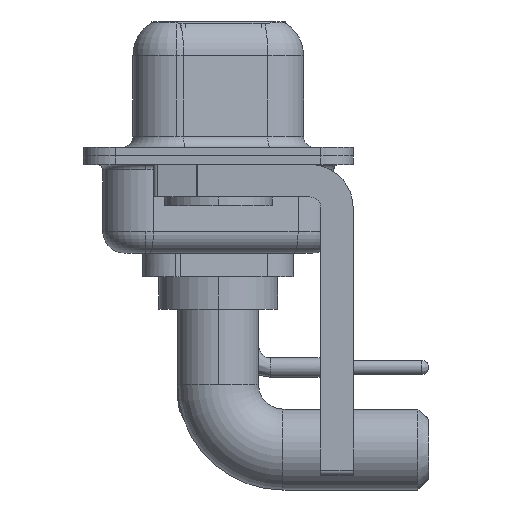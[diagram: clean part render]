
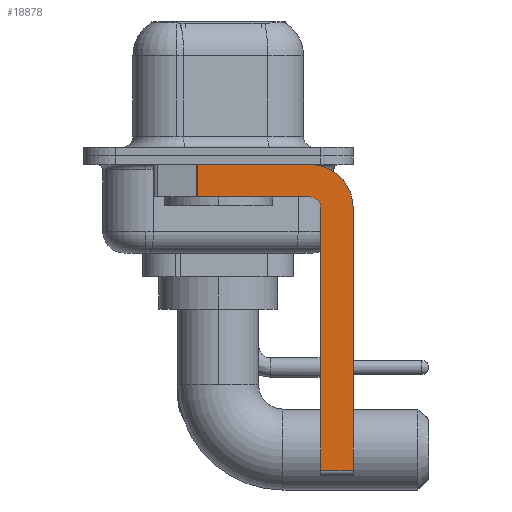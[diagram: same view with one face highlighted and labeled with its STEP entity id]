
A CAD part, left-side view. The second image highlights one B-rep face of the part: STEP entity #18878.
In plain terms, the highlighted planar face has unit normal (-1, 0, 0).
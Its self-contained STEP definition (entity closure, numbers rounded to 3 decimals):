
#360 = CARTESIAN_POINT ( 'NONE',  ( -2.9, -4.25, -0.4 ) ) ;
#599 = CARTESIAN_POINT ( 'NONE',  ( -2.9, -4.25, -1.9 ) ) ;
#852 = DIRECTION ( 'NONE',  ( 0., 0., 1. ) ) ;
#1183 = LINE ( 'NONE', #599, #2556 ) ;
#1853 = DIRECTION ( 'NONE',  ( 1., 0., 0. ) ) ;
#1893 = DIRECTION ( 'NONE',  ( -1., 0., 0. ) ) ;
#1949 = LINE ( 'NONE', #15132, #15423 ) ;
#2354 = EDGE_LOOP ( 'NONE', ( #16925, #16389, #22861, #15963, #22969, #20621, #24127, #7540 ) ) ;
#2556 = VECTOR ( 'NONE', #23903, 1000. ) ;
#2571 = VERTEX_POINT ( 'NONE', #15135 ) ;
#3588 = VECTOR ( 'NONE', #19046, 1000. ) ;
#4960 = VERTEX_POINT ( 'NONE', #17312 ) ;
#4984 = VERTEX_POINT ( 'NONE', #20901 ) ;
#5186 = LINE ( 'NONE', #14515, #7699 ) ;
#5392 = EDGE_CURVE ( 'NONE', #17463, #19019, #10856, .T. ) ;
#5721 = CARTESIAN_POINT ( 'NONE',  ( -2.9, -4.25, -2.4 ) ) ;
#5986 = EDGE_CURVE ( 'NONE', #4984, #2571, #1183, .T. ) ;
#6716 = CARTESIAN_POINT ( 'NONE',  ( -2.9, -4.25, -14.55 ) ) ;
#6918 = VERTEX_POINT ( 'NONE', #9969 ) ;
#7126 = DIRECTION ( 'NONE',  ( 0., -1., 0. ) ) ;
#7150 = CARTESIAN_POINT ( 'NONE',  ( -2.9, 0.978, -0.4 ) ) ;
#7217 = DIRECTION ( 'NONE',  ( 0., 0., -1. ) ) ;
#7540 = ORIENTED_EDGE ( 'NONE', *, *, #18860, .F. ) ;
#7699 = VECTOR ( 'NONE', #852, 1000. ) ;
#8272 = CARTESIAN_POINT ( 'NONE',  ( -2.9, -6.25, -14.55 ) ) ;
#8349 = DIRECTION ( 'NONE',  ( 0., -1., 0. ) ) ;
#9057 = CIRCLE ( 'NONE', #14216, 0.5 ) ;
#9092 = DIRECTION ( 'NONE',  ( 1., 0., 0. ) ) ;
#9969 = CARTESIAN_POINT ( 'NONE',  ( -2.9, -4.75, -14.55 ) ) ;
#10551 = EDGE_CURVE ( 'NONE', #6918, #4960, #5186, .T. ) ;
#10856 = LINE ( 'NONE', #24243, #21403 ) ;
#12441 = CARTESIAN_POINT ( 'NONE',  ( -2.9, -6.25, -2.4 ) ) ;
#13360 = CIRCLE ( 'NONE', #20479, 2. ) ;
#13542 = FACE_OUTER_BOUND ( 'NONE', #2354, .T. ) ;
#14216 = AXIS2_PLACEMENT_3D ( 'NONE', #22378, #1893, #20641 ) ;
#14515 = CARTESIAN_POINT ( 'NONE',  ( -2.9, -4.75, -14.8 ) ) ;
#14916 = DIRECTION ( 'NONE',  ( 0., 0., -1. ) ) ;
#15132 = CARTESIAN_POINT ( 'NONE',  ( -2.9, 0.978, -1.9 ) ) ;
#15135 = CARTESIAN_POINT ( 'NONE',  ( -2.9, 0.978, -1.9 ) ) ;
#15161 = PLANE ( 'NONE',  #18137 ) ;
#15423 = VECTOR ( 'NONE', #18736, 1000. ) ;
#15963 = ORIENTED_EDGE ( 'NONE', *, *, #20220, .F. ) ;
#16389 = ORIENTED_EDGE ( 'NONE', *, *, #21684, .T. ) ;
#16925 = ORIENTED_EDGE ( 'NONE', *, *, #5392, .F. ) ;
#17312 = CARTESIAN_POINT ( 'NONE',  ( -2.9, -4.75, -2.4 ) ) ;
#17463 = VERTEX_POINT ( 'NONE', #7150 ) ;
#18137 = AXIS2_PLACEMENT_3D ( 'NONE', #5721, #1853, #14916 ) ;
#18143 = LINE ( 'NONE', #6716, #18673 ) ;
#18410 = VERTEX_POINT ( 'NONE', #12441 ) ;
#18525 = CARTESIAN_POINT ( 'NONE',  ( -2.9, -4.25, -2.4 ) ) ;
#18673 = VECTOR ( 'NONE', #8349, 1000. ) ;
#18736 = DIRECTION ( 'NONE',  ( 0., 0., -1. ) ) ;
#18860 = EDGE_CURVE ( 'NONE', #19019, #18410, #13360, .T. ) ;
#18878 = ADVANCED_FACE ( 'NONE', ( #13542 ), #15161, .F. ) ;
#19019 = VERTEX_POINT ( 'NONE', #360 ) ;
#19046 = DIRECTION ( 'NONE',  ( 0., 0., -1. ) ) ;
#19175 = LINE ( 'NONE', #22384, #3588 ) ;
#20037 = VERTEX_POINT ( 'NONE', #8272 ) ;
#20220 = EDGE_CURVE ( 'NONE', #4960, #4984, #9057, .T. ) ;
#20479 = AXIS2_PLACEMENT_3D ( 'NONE', #18525, #9092, #7217 ) ;
#20621 = ORIENTED_EDGE ( 'NONE', *, *, #24048, .T. ) ;
#20641 = DIRECTION ( 'NONE',  ( 0., 0., 1. ) ) ;
#20901 = CARTESIAN_POINT ( 'NONE',  ( -2.9, -4.25, -1.9 ) ) ;
#21403 = VECTOR ( 'NONE', #7126, 1000. ) ;
#21684 = EDGE_CURVE ( 'NONE', #17463, #2571, #1949, .T. ) ;
#22378 = CARTESIAN_POINT ( 'NONE',  ( -2.9, -4.25, -2.4 ) ) ;
#22384 = CARTESIAN_POINT ( 'NONE',  ( -2.9, -6.25, -2.4 ) ) ;
#22861 = ORIENTED_EDGE ( 'NONE', *, *, #5986, .F. ) ;
#22969 = ORIENTED_EDGE ( 'NONE', *, *, #10551, .F. ) ;
#23903 = DIRECTION ( 'NONE',  ( 0., 1., 0. ) ) ;
#23914 = EDGE_CURVE ( 'NONE', #18410, #20037, #19175, .T. ) ;
#24048 = EDGE_CURVE ( 'NONE', #6918, #20037, #18143, .T. ) ;
#24127 = ORIENTED_EDGE ( 'NONE', *, *, #23914, .F. ) ;
#24243 = CARTESIAN_POINT ( 'NONE',  ( -2.9, 3., -0.4 ) ) ;
